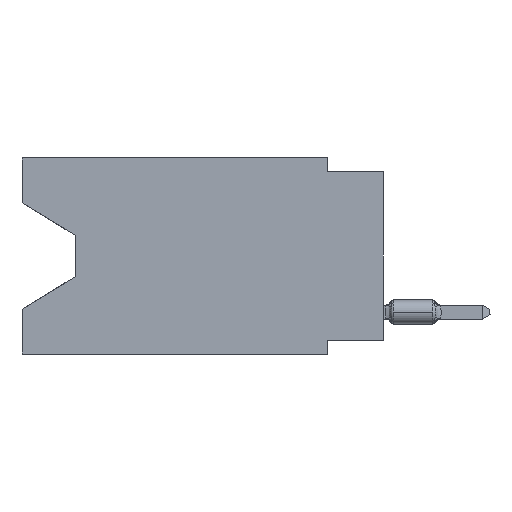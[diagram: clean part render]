
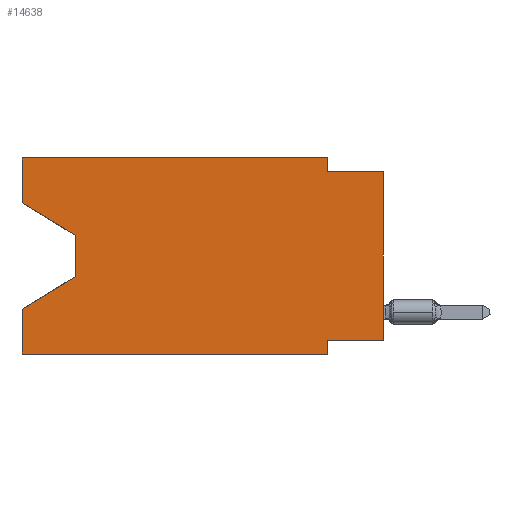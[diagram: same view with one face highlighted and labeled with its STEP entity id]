
A CAD part, left-side view. The second image highlights one B-rep face of the part: STEP entity #14638.
In plain terms, the highlighted planar face has unit normal (-1, 0, 0).
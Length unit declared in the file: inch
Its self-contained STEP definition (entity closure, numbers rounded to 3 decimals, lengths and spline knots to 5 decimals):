
#41 = DIRECTION ( 'NONE',  ( 1., 0., 0. ) ) ;
#348 = CARTESIAN_POINT ( 'NONE',  ( 0., 0., 0. ) ) ;
#718 = LINE ( 'NONE', #12149, #24448 ) ;
#725 = VECTOR ( 'NONE', #24738, 39.37008 ) ;
#976 = EDGE_CURVE ( 'NONE', #8899, #9215, #13300, .T. ) ;
#1014 = ORIENTED_EDGE ( 'NONE', *, *, #18486, .T. ) ;
#1901 = CARTESIAN_POINT ( 'NONE',  ( 0., 0.645, 0. ) ) ;
#2289 = ORIENTED_EDGE ( 'NONE', *, *, #976, .T. ) ;
#2447 = DIRECTION ( 'NONE',  ( 0., 0., 1. ) ) ;
#3830 = VECTOR ( 'NONE', #17674, 39.37008 ) ;
#4176 = LINE ( 'NONE', #11738, #21942 ) ;
#4286 = AXIS2_PLACEMENT_3D ( 'NONE', #1901, #41, #28275 ) ;
#4378 = EDGE_CURVE ( 'NONE', #29979, #21254, #19787, .T. ) ;
#4409 = CARTESIAN_POINT ( 'NONE',  ( 0., 0.1, -0.35 ) ) ;
#4627 = EDGE_CURVE ( 'NONE', #6186, #9215, #21845, .T. ) ;
#4807 = CARTESIAN_POINT ( 'NONE',  ( 0., 0.645, -0.08025 ) ) ;
#5599 = CARTESIAN_POINT ( 'NONE',  ( 0., 0.645, -0.35 ) ) ;
#5614 = VECTOR ( 'NONE', #20843, 39.37008 ) ;
#6124 = ORIENTED_EDGE ( 'NONE', *, *, #24161, .T. ) ;
#6186 = VERTEX_POINT ( 'NONE', #5599 ) ;
#6228 = CARTESIAN_POINT ( 'NONE',  ( 0., 0.55, -0.212 ) ) ;
#7187 = ORIENTED_EDGE ( 'NONE', *, *, #27941, .F. ) ;
#7354 = CARTESIAN_POINT ( 'NONE',  ( 0., 0.1, -0.325 ) ) ;
#7659 = CARTESIAN_POINT ( 'NONE',  ( 0., 0.1, 0. ) ) ;
#7813 = CARTESIAN_POINT ( 'NONE',  ( 0., 0.55, -0.138 ) ) ;
#8021 = ORIENTED_EDGE ( 'NONE', *, *, #4378, .F. ) ;
#8384 = DIRECTION ( 'NONE',  ( 0., 0.855, -0.519 ) ) ;
#8506 = CARTESIAN_POINT ( 'NONE',  ( 0., 0., -0.025 ) ) ;
#8697 = CARTESIAN_POINT ( 'NONE',  ( 0., 0.645, -0.35 ) ) ;
#8899 = VERTEX_POINT ( 'NONE', #20837 ) ;
#9215 = VERTEX_POINT ( 'NONE', #27599 ) ;
#9401 = VECTOR ( 'NONE', #23008, 39.37008 ) ;
#10102 = CARTESIAN_POINT ( 'NONE',  ( 0., 0.55, -0.138 ) ) ;
#10379 = DIRECTION ( 'NONE',  ( 0., 1., 0. ) ) ;
#11054 = VECTOR ( 'NONE', #17857, 39.37008 ) ;
#11438 = EDGE_CURVE ( 'NONE', #21254, #14632, #15976, .T. ) ;
#11588 = VERTEX_POINT ( 'NONE', #7813 ) ;
#11592 = VERTEX_POINT ( 'NONE', #7659 ) ;
#11738 = CARTESIAN_POINT ( 'NONE',  ( 0., 0.1, 0. ) ) ;
#11798 = VERTEX_POINT ( 'NONE', #4807 ) ;
#12093 = ORIENTED_EDGE ( 'NONE', *, *, #11438, .F. ) ;
#12149 = CARTESIAN_POINT ( 'NONE',  ( 0., 0.645, -0.08025 ) ) ;
#13300 = LINE ( 'NONE', #6228, #15860 ) ;
#14227 = VERTEX_POINT ( 'NONE', #21214 ) ;
#14632 = VERTEX_POINT ( 'NONE', #25347 ) ;
#14638 = ADVANCED_FACE ( 'NONE', ( #27982 ), #15930, .F. ) ;
#15125 = ORIENTED_EDGE ( 'NONE', *, *, #27193, .T. ) ;
#15174 = ORIENTED_EDGE ( 'NONE', *, *, #30029, .F. ) ;
#15230 = CARTESIAN_POINT ( 'NONE',  ( 0., 0., -0.025 ) ) ;
#15679 = CARTESIAN_POINT ( 'NONE',  ( 0., 0.1, -0.025 ) ) ;
#15685 = LINE ( 'NONE', #15230, #11054 ) ;
#15860 = VECTOR ( 'NONE', #8384, 39.37008 ) ;
#15925 = VECTOR ( 'NONE', #20621, 39.37008 ) ;
#15930 = PLANE ( 'NONE',  #4286 ) ;
#15976 = LINE ( 'NONE', #4409, #15925 ) ;
#16663 = EDGE_CURVE ( 'NONE', #14227, #11592, #23301, .T. ) ;
#17011 = VECTOR ( 'NONE', #2447, 39.37008 ) ;
#17059 = DIRECTION ( 'NONE',  ( 0., 0., -1. ) ) ;
#17337 = LINE ( 'NONE', #10102, #21462 ) ;
#17486 = CARTESIAN_POINT ( 'NONE',  ( 0., 0., -0.325 ) ) ;
#17674 = DIRECTION ( 'NONE',  ( 0., 0., 1. ) ) ;
#17857 = DIRECTION ( 'NONE',  ( 0., -1., 0. ) ) ;
#18486 = EDGE_CURVE ( 'NONE', #6186, #14632, #22268, .T. ) ;
#18607 = VECTOR ( 'NONE', #10379, 39.37008 ) ;
#18834 = LINE ( 'NONE', #348, #5614 ) ;
#19091 = DIRECTION ( 'NONE',  ( 0., -0.855, -0.519 ) ) ;
#19641 = EDGE_CURVE ( 'NONE', #11588, #8899, #17337, .T. ) ;
#19787 = LINE ( 'NONE', #17486, #18607 ) ;
#20541 = CARTESIAN_POINT ( 'NONE',  ( 0., 0.645, 0. ) ) ;
#20621 = DIRECTION ( 'NONE',  ( 0., 0., -1. ) ) ;
#20790 = EDGE_CURVE ( 'NONE', #11592, #26789, #4176, .T. ) ;
#20837 = CARTESIAN_POINT ( 'NONE',  ( 0., 0.55, -0.212 ) ) ;
#20842 = ORIENTED_EDGE ( 'NONE', *, *, #20790, .F. ) ;
#20843 = DIRECTION ( 'NONE',  ( 0., 0., 1. ) ) ;
#21170 = ORIENTED_EDGE ( 'NONE', *, *, #16663, .F. ) ;
#21214 = CARTESIAN_POINT ( 'NONE',  ( 0., 0.645, 0. ) ) ;
#21254 = VERTEX_POINT ( 'NONE', #7354 ) ;
#21462 = VECTOR ( 'NONE', #17059, 39.37008 ) ;
#21845 = LINE ( 'NONE', #22454, #3830 ) ;
#21942 = VECTOR ( 'NONE', #25782, 39.37008 ) ;
#22067 = ORIENTED_EDGE ( 'NONE', *, *, #19641, .T. ) ;
#22268 = LINE ( 'NONE', #8697, #725 ) ;
#22454 = CARTESIAN_POINT ( 'NONE',  ( 0., 0.645, 0. ) ) ;
#22833 = ORIENTED_EDGE ( 'NONE', *, *, #4627, .F. ) ;
#22992 = CARTESIAN_POINT ( 'NONE',  ( 0., 0., -0.325 ) ) ;
#23008 = DIRECTION ( 'NONE',  ( 0., -1., 0. ) ) ;
#23301 = LINE ( 'NONE', #20541, #9401 ) ;
#23454 = CARTESIAN_POINT ( 'NONE',  ( 0., 0.645, 0. ) ) ;
#23668 = EDGE_LOOP ( 'NONE', ( #6124, #22067, #2289, #22833, #1014, #12093, #8021, #15125, #7187, #20842, #21170, #15174 ) ) ;
#24161 = EDGE_CURVE ( 'NONE', #11798, #11588, #718, .T. ) ;
#24448 = VECTOR ( 'NONE', #19091, 39.37008 ) ;
#24738 = DIRECTION ( 'NONE',  ( 0., -1., 0. ) ) ;
#25347 = CARTESIAN_POINT ( 'NONE',  ( 0., 0.1, -0.35 ) ) ;
#25782 = DIRECTION ( 'NONE',  ( 0., 0., -1. ) ) ;
#26001 = VERTEX_POINT ( 'NONE', #8506 ) ;
#26789 = VERTEX_POINT ( 'NONE', #15679 ) ;
#27193 = EDGE_CURVE ( 'NONE', #29979, #26001, #18834, .T. ) ;
#27599 = CARTESIAN_POINT ( 'NONE',  ( 0., 0.645, -0.26975 ) ) ;
#27941 = EDGE_CURVE ( 'NONE', #26789, #26001, #15685, .T. ) ;
#27982 = FACE_OUTER_BOUND ( 'NONE', #23668, .T. ) ;
#28275 = DIRECTION ( 'NONE',  ( 0., 0., -1. ) ) ;
#28535 = LINE ( 'NONE', #23454, #17011 ) ;
#29979 = VERTEX_POINT ( 'NONE', #22992 ) ;
#30029 = EDGE_CURVE ( 'NONE', #11798, #14227, #28535, .T. ) ;
